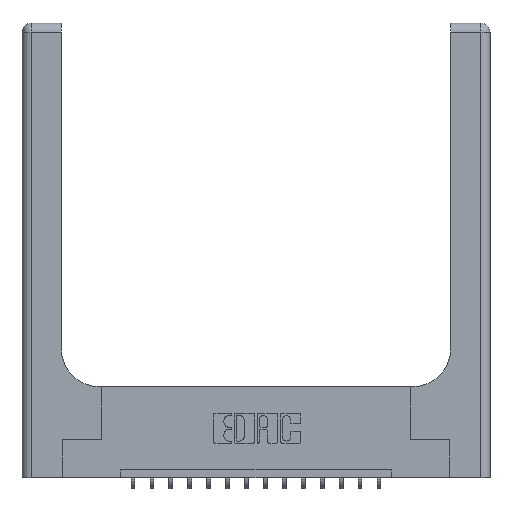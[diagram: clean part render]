
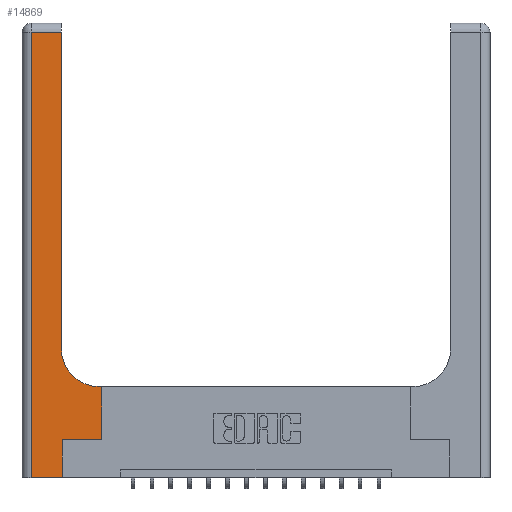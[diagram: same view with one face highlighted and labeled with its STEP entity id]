
A CAD part, top view. The second image highlights one B-rep face of the part: STEP entity #14869.
In plain terms, the highlighted planar face has unit normal (0, 0, 1).
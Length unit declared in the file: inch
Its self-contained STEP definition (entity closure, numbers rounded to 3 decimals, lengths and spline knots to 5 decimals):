
#234 = DIRECTION ( 'NONE',  ( 0., 1., 0. ) ) ;
#369 = CIRCLE ( 'NONE', #13593, 0.25 ) ;
#386 = CARTESIAN_POINT ( 'NONE',  ( 0.26, 0.6, 0.37 ) ) ;
#620 = EDGE_LOOP ( 'NONE', ( #6559, #3342, #5295, #2573, #3301, #13285, #12385, #1354, #11708 ) ) ;
#835 = DIRECTION ( 'NONE',  ( 0., 1., 0. ) ) ;
#855 = CARTESIAN_POINT ( 'NONE',  ( 0.26, 0.85, 0.37 ) ) ;
#1138 = DIRECTION ( 'NONE',  ( 0., 1., 0. ) ) ;
#1181 = DIRECTION ( 'NONE',  ( -1., 0., 0. ) ) ;
#1354 = ORIENTED_EDGE ( 'NONE', *, *, #17590, .T. ) ;
#1430 = DIRECTION ( 'NONE',  ( -1., 0., 0. ) ) ;
#1594 = VECTOR ( 'NONE', #17045, 39.37008 ) ;
#1597 = EDGE_CURVE ( 'NONE', #6259, #8591, #16808, .T. ) ;
#1642 = EDGE_CURVE ( 'NONE', #7811, #8313, #15973, .T. ) ;
#1785 = DIRECTION ( 'NONE',  ( -1., 0., 0. ) ) ;
#2100 = EDGE_CURVE ( 'NONE', #8591, #7811, #10562, .T. ) ;
#2573 = ORIENTED_EDGE ( 'NONE', *, *, #1597, .T. ) ;
#2691 = VECTOR ( 'NONE', #835, 39.37008 ) ;
#2924 = VECTOR ( 'NONE', #1138, 39.37008 ) ;
#3301 = ORIENTED_EDGE ( 'NONE', *, *, #2100, .T. ) ;
#3342 = ORIENTED_EDGE ( 'NONE', *, *, #14756, .T. ) ;
#3356 = VECTOR ( 'NONE', #1785, 39.37008 ) ;
#4141 = CARTESIAN_POINT ( 'NONE',  ( 0., 3., 0.37 ) ) ;
#4395 = CARTESIAN_POINT ( 'NONE',  ( 0.528, 0.25, 0.37 ) ) ;
#4728 = CARTESIAN_POINT ( 'NONE',  ( 0.26, 2.94, 0.37 ) ) ;
#4898 = CARTESIAN_POINT ( 'NONE',  ( 0.06, 3., 0.37 ) ) ;
#5295 = ORIENTED_EDGE ( 'NONE', *, *, #11531, .T. ) ;
#6259 = VERTEX_POINT ( 'NONE', #8553 ) ;
#6531 = CARTESIAN_POINT ( 'NONE',  ( 0.265, 0.25, 0.37 ) ) ;
#6559 = ORIENTED_EDGE ( 'NONE', *, *, #9316, .T. ) ;
#7046 = EDGE_CURVE ( 'NONE', #17609, #12746, #369, .T. ) ;
#7075 = CARTESIAN_POINT ( 'NONE',  ( 0., 0., 0.37 ) ) ;
#7630 = CARTESIAN_POINT ( 'NONE',  ( 0.51, 0.85, 0.37 ) ) ;
#7811 = VERTEX_POINT ( 'NONE', #15496 ) ;
#8021 = FACE_OUTER_BOUND ( 'NONE', #620, .T. ) ;
#8104 = CARTESIAN_POINT ( 'NONE',  ( 0.26, 3., 0.37 ) ) ;
#8313 = VERTEX_POINT ( 'NONE', #16832 ) ;
#8357 = VERTEX_POINT ( 'NONE', #4728 ) ;
#8553 = CARTESIAN_POINT ( 'NONE',  ( 0.06, 0., 0.37 ) ) ;
#8591 = VERTEX_POINT ( 'NONE', #10732 ) ;
#9007 = DIRECTION ( 'NONE',  ( 1., 0., 0. ) ) ;
#9018 = LINE ( 'NONE', #4898, #1594 ) ;
#9145 = VERTEX_POINT ( 'NONE', #14531 ) ;
#9316 = EDGE_CURVE ( 'NONE', #12746, #8357, #13910, .T. ) ;
#9535 = CARTESIAN_POINT ( 'NONE',  ( 0., 2.94, 0.37 ) ) ;
#9781 = DIRECTION ( 'NONE',  ( 0., 0., -1. ) ) ;
#9817 = DIRECTION ( 'NONE',  ( 1., 0., 0. ) ) ;
#9975 = VECTOR ( 'NONE', #234, 39.37008 ) ;
#10209 = VECTOR ( 'NONE', #1181, 39.37008 ) ;
#10317 = AXIS2_PLACEMENT_3D ( 'NONE', #4141, #9781, #1430 ) ;
#10562 = LINE ( 'NONE', #15948, #2691 ) ;
#10732 = CARTESIAN_POINT ( 'NONE',  ( 0.265, 0., 0.37 ) ) ;
#10761 = LINE ( 'NONE', #386, #3356 ) ;
#11531 = EDGE_CURVE ( 'NONE', #9145, #6259, #9018, .T. ) ;
#11599 = CARTESIAN_POINT ( 'NONE',  ( 0.528, 0.6, 0.37 ) ) ;
#11708 = ORIENTED_EDGE ( 'NONE', *, *, #7046, .T. ) ;
#12385 = ORIENTED_EDGE ( 'NONE', *, *, #14973, .T. ) ;
#12470 = VECTOR ( 'NONE', #17412, 39.37008 ) ;
#12746 = VERTEX_POINT ( 'NONE', #855 ) ;
#13272 = VECTOR ( 'NONE', #9817, 39.37008 ) ;
#13285 = ORIENTED_EDGE ( 'NONE', *, *, #1642, .T. ) ;
#13593 = AXIS2_PLACEMENT_3D ( 'NONE', #7630, #17016, #9007 ) ;
#13910 = LINE ( 'NONE', #8104, #2924 ) ;
#14220 = CARTESIAN_POINT ( 'NONE',  ( 0.51, 0.6, 0.37 ) ) ;
#14531 = CARTESIAN_POINT ( 'NONE',  ( 0.06, 2.94, 0.37 ) ) ;
#14756 = EDGE_CURVE ( 'NONE', #8357, #9145, #17249, .T. ) ;
#14869 = ADVANCED_FACE ( 'NONE', ( #8021 ), #16430, .F. ) ;
#14973 = EDGE_CURVE ( 'NONE', #8313, #17189, #17051, .T. ) ;
#15496 = CARTESIAN_POINT ( 'NONE',  ( 0.265, 0.25, 0.37 ) ) ;
#15948 = CARTESIAN_POINT ( 'NONE',  ( 0.265, 0., 0.37 ) ) ;
#15973 = LINE ( 'NONE', #6531, #12470 ) ;
#16430 = PLANE ( 'NONE',  #10317 ) ;
#16808 = LINE ( 'NONE', #7075, #13272 ) ;
#16832 = CARTESIAN_POINT ( 'NONE',  ( 0.528, 0.25, 0.37 ) ) ;
#17016 = DIRECTION ( 'NONE',  ( 0., 0., -1. ) ) ;
#17045 = DIRECTION ( 'NONE',  ( 0., -1., 0. ) ) ;
#17051 = LINE ( 'NONE', #4395, #9975 ) ;
#17189 = VERTEX_POINT ( 'NONE', #11599 ) ;
#17249 = LINE ( 'NONE', #9535, #10209 ) ;
#17412 = DIRECTION ( 'NONE',  ( 1., 0., 0. ) ) ;
#17590 = EDGE_CURVE ( 'NONE', #17189, #17609, #10761, .T. ) ;
#17609 = VERTEX_POINT ( 'NONE', #14220 ) ;
